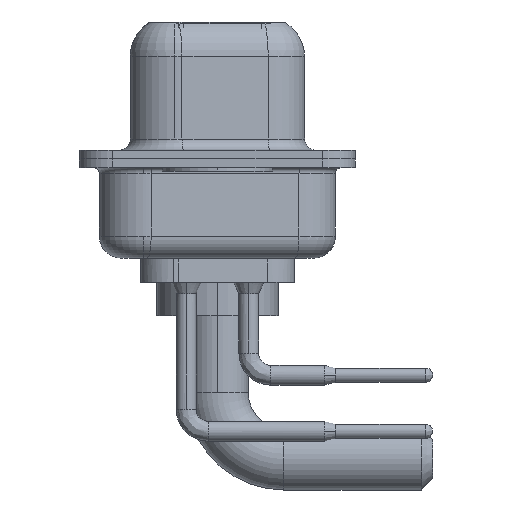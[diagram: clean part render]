
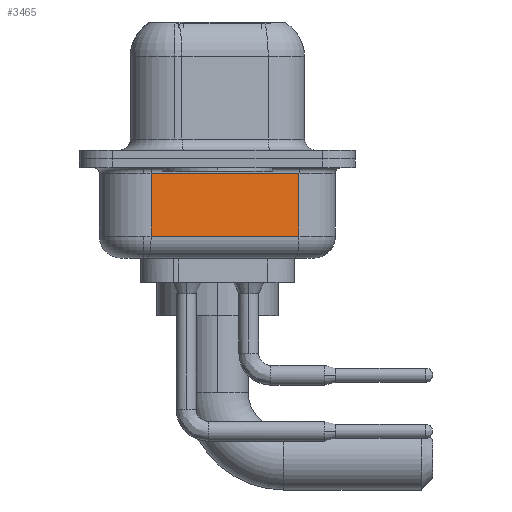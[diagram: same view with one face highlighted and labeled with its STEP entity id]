
A CAD part, left-side view. The second image highlights one B-rep face of the part: STEP entity #3465.
In plain terms, the highlighted planar face has unit normal (-0.985, -0.174, 0).
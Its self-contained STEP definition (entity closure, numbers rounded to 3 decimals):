
#450 = DIRECTION ( 'NONE',  ( 0., 0., 1. ) ) ;
#925 = VERTEX_POINT ( 'NONE', #12468 ) ;
#933 = AXIS2_PLACEMENT_3D ( 'NONE', #6953, #14969, #9658 ) ;
#1068 = EDGE_CURVE ( 'NONE', #15725, #925, #1156, .T. ) ;
#1156 = LINE ( 'NONE', #15459, #5072 ) ;
#1283 = CARTESIAN_POINT ( 'NONE',  ( 2.88, 3.003, -3.5 ) ) ;
#1873 = CARTESIAN_POINT ( 'NONE',  ( 4.062, -3.697, -4.5 ) ) ;
#2184 = VERTEX_POINT ( 'NONE', #12403 ) ;
#2448 = VECTOR ( 'NONE', #450, 1000. ) ;
#3154 = EDGE_CURVE ( 'NONE', #15725, #7829, #4813, .T. ) ;
#3465 = ADVANCED_FACE ( 'NONE', ( #14889 ), #9811, .F. ) ;
#3710 = ORIENTED_EDGE ( 'NONE', *, *, #14557, .T. ) ;
#3720 = EDGE_LOOP ( 'NONE', ( #4806, #12294, #9174, #3710 ) ) ;
#4540 = DIRECTION ( 'NONE',  ( -0.174, 0.985, 0. ) ) ;
#4800 = EDGE_CURVE ( 'NONE', #925, #2184, #11929, .T. ) ;
#4806 = ORIENTED_EDGE ( 'NONE', *, *, #3154, .F. ) ;
#4813 = LINE ( 'NONE', #10017, #13252 ) ;
#4930 = DIRECTION ( 'NONE',  ( 0.174, -0.985, 0. ) ) ;
#5072 = VECTOR ( 'NONE', #4930, 1000. ) ;
#5704 = LINE ( 'NONE', #10830, #8385 ) ;
#6953 = CARTESIAN_POINT ( 'NONE',  ( 2.88, 3.003, -4.5 ) ) ;
#7829 = VERTEX_POINT ( 'NONE', #16265 ) ;
#8385 = VECTOR ( 'NONE', #4540, 1000. ) ;
#9174 = ORIENTED_EDGE ( 'NONE', *, *, #4800, .T. ) ;
#9658 = DIRECTION ( 'NONE',  ( -0.174, 0.985, 0. ) ) ;
#9811 = PLANE ( 'NONE',  #933 ) ;
#10017 = CARTESIAN_POINT ( 'NONE',  ( 2.88, 3.003, -4.5 ) ) ;
#10830 = CARTESIAN_POINT ( 'NONE',  ( 2.88, 3.003, -0.65 ) ) ;
#11929 = LINE ( 'NONE', #1873, #2448 ) ;
#12294 = ORIENTED_EDGE ( 'NONE', *, *, #1068, .T. ) ;
#12403 = CARTESIAN_POINT ( 'NONE',  ( 4.062, -3.697, -0.65 ) ) ;
#12468 = CARTESIAN_POINT ( 'NONE',  ( 4.062, -3.697, -3.5 ) ) ;
#13252 = VECTOR ( 'NONE', #15176, 1000. ) ;
#14557 = EDGE_CURVE ( 'NONE', #2184, #7829, #5704, .T. ) ;
#14889 = FACE_OUTER_BOUND ( 'NONE', #3720, .T. ) ;
#14969 = DIRECTION ( 'NONE',  ( 0.985, 0.174, 0. ) ) ;
#15176 = DIRECTION ( 'NONE',  ( 0., 0., 1. ) ) ;
#15459 = CARTESIAN_POINT ( 'NONE',  ( 2.88, 3.003, -3.5 ) ) ;
#15725 = VERTEX_POINT ( 'NONE', #1283 ) ;
#16265 = CARTESIAN_POINT ( 'NONE',  ( 2.88, 3.003, -0.65 ) ) ;
